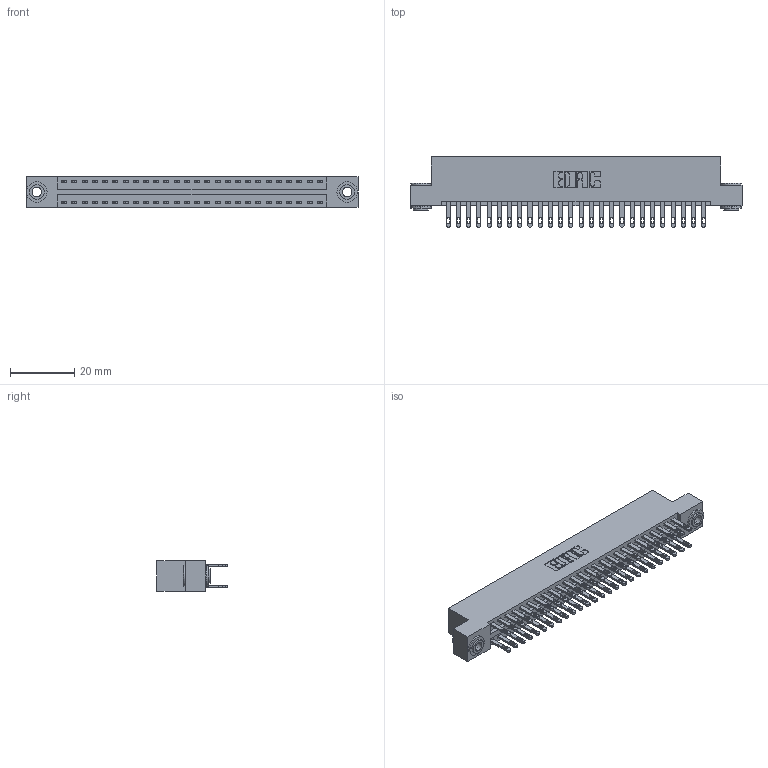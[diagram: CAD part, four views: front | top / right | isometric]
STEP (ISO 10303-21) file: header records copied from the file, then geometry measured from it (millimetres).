
FILE_DESCRIPTION (( 'STEP AP203' ), '1' );
FILE_NAME ('346-052-500-203.STEP', '2018-08-27T23:22:05', ( '' ), ( '' ), 'SwSTEP 2.0', 'SolidWorks 2016', '' );
FILE_SCHEMA (( 'CONFIG_CONTROL_DESIGN' ));
Length unit declared in the file: inch
Products named in the file (4): 345-250-002_345-250-002-102; 346-052-500-203; 346 Part_Flush Mounting Lugs - 0.156 Dia-TH; 345-292-001_345-293-100
Assembly tree (55 placements, depth 2):
  346-052-500-203
    346 Part_Flush Mounting Lugs - 0.156 Dia-TH
    345-292-001_345-293-100  x52
    345-250-002_345-250-002-102  x2
Bounding box: 103.12 x 21.84 x 9.4 mm (x, y, z)
Volume: 10109.9 mm3; surface area: 14403.7 mm2
Topology: 55 solids, 55 shells, 2656 faces, 8049 edges, 5362 vertices
Faces by surface type: plane 1594, cylinder 1054, cone 8
Entity records: 19702 total; most frequent: CARTESIAN_POINT 3243, ORIENTED_EDGE 3170, DIRECTION 2943, EDGE_CURVE 1585, LINE 1321, VECTOR 1321, VERTEX_POINT 1054, AXIS2_PLACEMENT_3D 811
